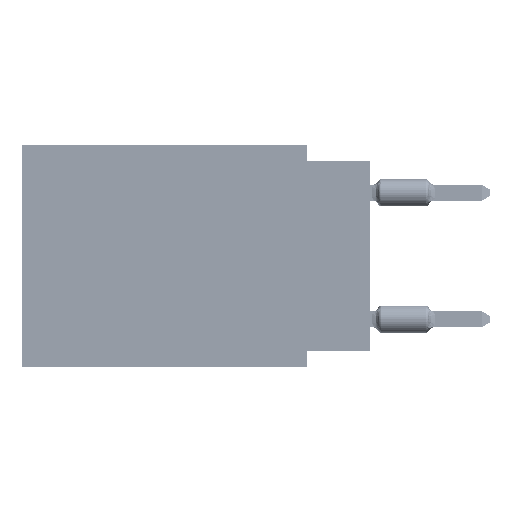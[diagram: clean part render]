
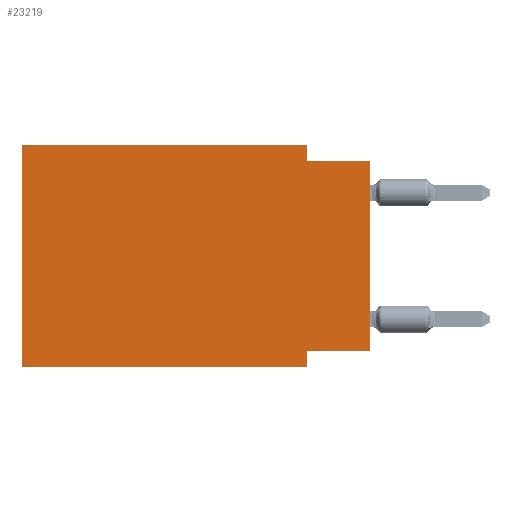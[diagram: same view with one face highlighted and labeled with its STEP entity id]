
A CAD part, left-side view. The second image highlights one B-rep face of the part: STEP entity #23219.
In plain terms, the highlighted planar face has unit normal (-1, 0, 0).
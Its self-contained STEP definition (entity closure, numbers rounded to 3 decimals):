
#1005 = DIRECTION ( 'NONE',  ( 0., -1., 0. ) ) ;
#1101 = VERTEX_POINT ( 'NONE', #38765 ) ;
#1381 = VECTOR ( 'NONE', #4986, 1000. ) ;
#3217 = ORIENTED_EDGE ( 'NONE', *, *, #56702, .F. ) ;
#3456 = ORIENTED_EDGE ( 'NONE', *, *, #20394, .T. ) ;
#3936 = LINE ( 'NONE', #19777, #22639 ) ;
#4808 = CARTESIAN_POINT ( 'NONE',  ( 0., 2.54, 0. ) ) ;
#4986 = DIRECTION ( 'NONE',  ( 0., 0., 1. ) ) ;
#6925 = CARTESIAN_POINT ( 'NONE',  ( 0., 2.54, -8.89 ) ) ;
#9219 = LINE ( 'NONE', #6925, #19746 ) ;
#9461 = VERTEX_POINT ( 'NONE', #36065 ) ;
#9642 = AXIS2_PLACEMENT_3D ( 'NONE', #11899, #66378, #38334 ) ;
#11072 = DIRECTION ( 'NONE',  ( 0., 1., 0. ) ) ;
#11899 = CARTESIAN_POINT ( 'NONE',  ( 0., 13.97, 0. ) ) ;
#13590 = VERTEX_POINT ( 'NONE', #66916 ) ;
#15128 = VECTOR ( 'NONE', #33499, 1000. ) ;
#15407 = CARTESIAN_POINT ( 'NONE',  ( 0., 2.54, -8.255 ) ) ;
#16832 = CARTESIAN_POINT ( 'NONE',  ( 0., 0., -0.635 ) ) ;
#17003 = EDGE_CURVE ( 'NONE', #9461, #25457, #58119, .T. ) ;
#18521 = VECTOR ( 'NONE', #1005, 1000. ) ;
#19746 = VECTOR ( 'NONE', #40487, 1000. ) ;
#19777 = CARTESIAN_POINT ( 'NONE',  ( 0., 2.54, 0. ) ) ;
#20394 = EDGE_CURVE ( 'NONE', #47514, #52104, #65338, .T. ) ;
#20885 = ORIENTED_EDGE ( 'NONE', *, *, #23282, .T. ) ;
#22639 = VECTOR ( 'NONE', #51329, 1000. ) ;
#23014 = VECTOR ( 'NONE', #60215, 1000. ) ;
#23219 = ADVANCED_FACE ( 'NONE', ( #48956 ), #65097, .F. ) ;
#23282 = EDGE_CURVE ( 'NONE', #9461, #1101, #38656, .T. ) ;
#24024 = EDGE_CURVE ( 'NONE', #13590, #51529, #64180, .T. ) ;
#25457 = VERTEX_POINT ( 'NONE', #15407 ) ;
#26185 = CARTESIAN_POINT ( 'NONE',  ( 0., 0., -8.255 ) ) ;
#27100 = CARTESIAN_POINT ( 'NONE',  ( 0., 13.97, 0. ) ) ;
#27821 = CARTESIAN_POINT ( 'NONE',  ( 0., 13.97, -8.89 ) ) ;
#31405 = EDGE_CURVE ( 'NONE', #66008, #1101, #63568, .T. ) ;
#32455 = ORIENTED_EDGE ( 'NONE', *, *, #31405, .F. ) ;
#33499 = DIRECTION ( 'NONE',  ( 0., 0., 1. ) ) ;
#33703 = EDGE_CURVE ( 'NONE', #51529, #66008, #3936, .T. ) ;
#36065 = CARTESIAN_POINT ( 'NONE',  ( 0., 0., -8.255 ) ) ;
#37926 = ORIENTED_EDGE ( 'NONE', *, *, #43232, .F. ) ;
#38334 = DIRECTION ( 'NONE',  ( 0., 0., -1. ) ) ;
#38656 = LINE ( 'NONE', #56102, #15128 ) ;
#38765 = CARTESIAN_POINT ( 'NONE',  ( 0., 0., -0.635 ) ) ;
#39241 = CARTESIAN_POINT ( 'NONE',  ( 0., 13.97, -8.89 ) ) ;
#40487 = DIRECTION ( 'NONE',  ( 0., 0., -1. ) ) ;
#41921 = DIRECTION ( 'NONE',  ( 0., -1., 0. ) ) ;
#42071 = CARTESIAN_POINT ( 'NONE',  ( 0., 13.97, 0. ) ) ;
#43232 = EDGE_CURVE ( 'NONE', #25457, #52104, #9219, .T. ) ;
#43701 = ORIENTED_EDGE ( 'NONE', *, *, #33703, .F. ) ;
#44249 = VECTOR ( 'NONE', #11072, 1000. ) ;
#45680 = ORIENTED_EDGE ( 'NONE', *, *, #17003, .F. ) ;
#46055 = VECTOR ( 'NONE', #41921, 1000. ) ;
#46312 = ORIENTED_EDGE ( 'NONE', *, *, #24024, .F. ) ;
#47514 = VERTEX_POINT ( 'NONE', #27821 ) ;
#48956 = FACE_OUTER_BOUND ( 'NONE', #59642, .T. ) ;
#51329 = DIRECTION ( 'NONE',  ( 0., 0., -1. ) ) ;
#51529 = VERTEX_POINT ( 'NONE', #4808 ) ;
#52104 = VERTEX_POINT ( 'NONE', #60347 ) ;
#56102 = CARTESIAN_POINT ( 'NONE',  ( 0., 0., 0. ) ) ;
#56702 = EDGE_CURVE ( 'NONE', #47514, #13590, #57540, .T. ) ;
#56825 = CARTESIAN_POINT ( 'NONE',  ( 0., 2.54, -0.635 ) ) ;
#57540 = LINE ( 'NONE', #42071, #1381 ) ;
#58119 = LINE ( 'NONE', #26185, #44249 ) ;
#59642 = EDGE_LOOP ( 'NONE', ( #20885, #32455, #43701, #46312, #3217, #3456, #37926, #45680 ) ) ;
#60215 = DIRECTION ( 'NONE',  ( 0., -1., 0. ) ) ;
#60347 = CARTESIAN_POINT ( 'NONE',  ( 0., 2.54, -8.89 ) ) ;
#63568 = LINE ( 'NONE', #16832, #46055 ) ;
#64180 = LINE ( 'NONE', #27100, #18521 ) ;
#65097 = PLANE ( 'NONE',  #9642 ) ;
#65338 = LINE ( 'NONE', #39241, #23014 ) ;
#66008 = VERTEX_POINT ( 'NONE', #56825 ) ;
#66378 = DIRECTION ( 'NONE',  ( 1., 0., 0. ) ) ;
#66916 = CARTESIAN_POINT ( 'NONE',  ( 0., 13.97, 0. ) ) ;
